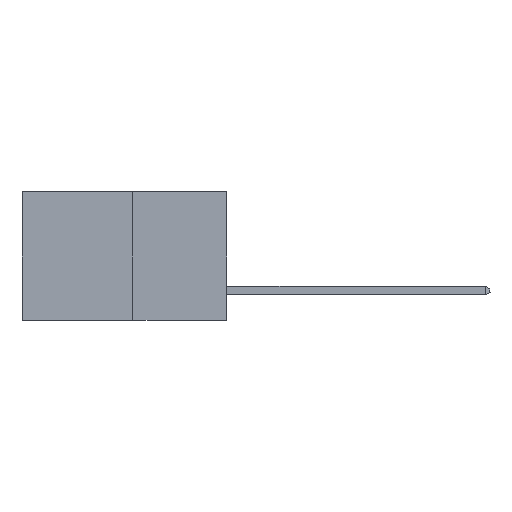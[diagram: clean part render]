
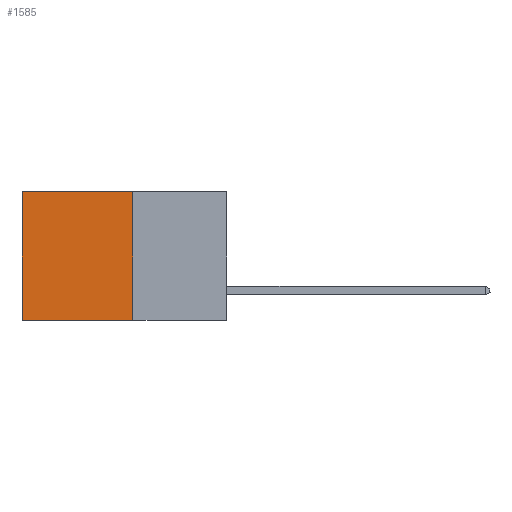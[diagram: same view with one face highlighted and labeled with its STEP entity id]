
A CAD part, left-side view. The second image highlights one B-rep face of the part: STEP entity #1585.
In plain terms, the highlighted planar face has unit normal (-1, 0, 0).
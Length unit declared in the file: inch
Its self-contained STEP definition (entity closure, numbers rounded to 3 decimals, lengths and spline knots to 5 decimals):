
#928 = CARTESIAN_POINT ( 'NONE',  ( 0.277, 0.27, 0. ) ) ;
#953 = VECTOR ( 'NONE', #23250, 39.37008 ) ;
#1071 = LINE ( 'NONE', #8562, #21802 ) ;
#1585 = ADVANCED_FACE ( 'NONE', ( #23930 ), #24512, .F. ) ;
#1658 = ORIENTED_EDGE ( 'NONE', *, *, #10598, .F. ) ;
#2064 = CARTESIAN_POINT ( 'NONE',  ( 0.277, 0.59, 0. ) ) ;
#2442 = LINE ( 'NONE', #8206, #12879 ) ;
#2455 = VERTEX_POINT ( 'NONE', #928 ) ;
#5683 = CARTESIAN_POINT ( 'NONE',  ( 0.277, 0.59, -0.37 ) ) ;
#6195 = VERTEX_POINT ( 'NONE', #20037 ) ;
#6807 = LINE ( 'NONE', #5683, #12539 ) ;
#7591 = LINE ( 'NONE', #17433, #953 ) ;
#8206 = CARTESIAN_POINT ( 'NONE',  ( 0.277, 0.27, -0.37 ) ) ;
#8562 = CARTESIAN_POINT ( 'NONE',  ( 0.277, 0.27, 0. ) ) ;
#10598 = EDGE_CURVE ( 'NONE', #16602, #6195, #2442, .T. ) ;
#10869 = ORIENTED_EDGE ( 'NONE', *, *, #17615, .T. ) ;
#12196 = ORIENTED_EDGE ( 'NONE', *, *, #14606, .F. ) ;
#12539 = VECTOR ( 'NONE', #17227, 39.37008 ) ;
#12879 = VECTOR ( 'NONE', #21602, 39.37008 ) ;
#14606 = EDGE_CURVE ( 'NONE', #2455, #16602, #7591, .T. ) ;
#15283 = AXIS2_PLACEMENT_3D ( 'NONE', #24256, #24233, #24202 ) ;
#16134 = DIRECTION ( 'NONE',  ( 0., 1., 0. ) ) ;
#16602 = VERTEX_POINT ( 'NONE', #21571 ) ;
#17227 = DIRECTION ( 'NONE',  ( 0., 0., -1. ) ) ;
#17433 = CARTESIAN_POINT ( 'NONE',  ( 0.277, 0.27, -0.37 ) ) ;
#17615 = EDGE_CURVE ( 'NONE', #21709, #6195, #6807, .T. ) ;
#20037 = CARTESIAN_POINT ( 'NONE',  ( 0.277, 0.59, -0.37 ) ) ;
#20831 = EDGE_LOOP ( 'NONE', ( #10869, #1658, #12196, #23819 ) ) ;
#21571 = CARTESIAN_POINT ( 'NONE',  ( 0.277, 0.27, -0.37 ) ) ;
#21602 = DIRECTION ( 'NONE',  ( 0., 1., 0. ) ) ;
#21709 = VERTEX_POINT ( 'NONE', #2064 ) ;
#21802 = VECTOR ( 'NONE', #16134, 39.37008 ) ;
#23250 = DIRECTION ( 'NONE',  ( 0., 0., -1. ) ) ;
#23752 = EDGE_CURVE ( 'NONE', #2455, #21709, #1071, .T. ) ;
#23819 = ORIENTED_EDGE ( 'NONE', *, *, #23752, .T. ) ;
#23930 = FACE_OUTER_BOUND ( 'NONE', #20831, .T. ) ;
#24202 = DIRECTION ( 'NONE',  ( 0., 0., -1. ) ) ;
#24233 = DIRECTION ( 'NONE',  ( 1., 0., 0. ) ) ;
#24256 = CARTESIAN_POINT ( 'NONE',  ( 0.277, 0.27, -0.37 ) ) ;
#24512 = PLANE ( 'NONE',  #15283 ) ;
